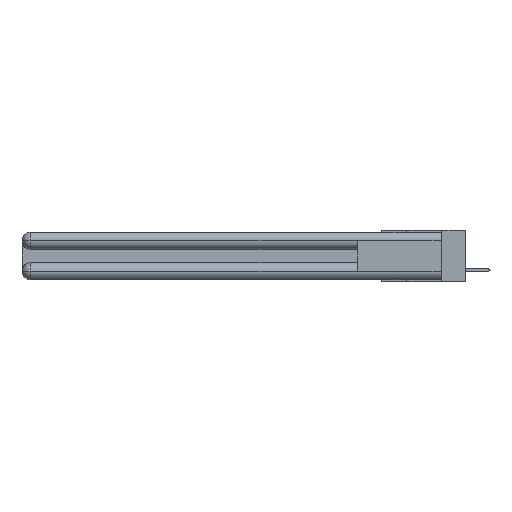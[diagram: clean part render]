
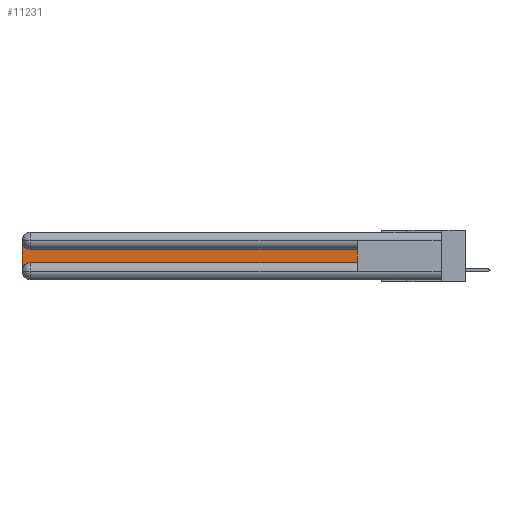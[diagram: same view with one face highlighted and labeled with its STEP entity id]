
A CAD part, left-side view. The second image highlights one B-rep face of the part: STEP entity #11231.
In plain terms, the highlighted planar face has unit normal (-1, 0, 0).
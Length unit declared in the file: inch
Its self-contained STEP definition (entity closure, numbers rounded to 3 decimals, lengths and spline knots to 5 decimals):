
#321 = ORIENTED_EDGE ( 'NONE', *, *, #31516, .T. ) ;
#532 = CARTESIAN_POINT ( 'NONE',  ( 0.075, 2.94, -0.0625 ) ) ;
#1027 = EDGE_CURVE ( 'NONE', #16137, #26790, #10930, .T. ) ;
#1420 = DIRECTION ( 'NONE',  ( 0., 1., 0. ) ) ;
#3016 = ORIENTED_EDGE ( 'NONE', *, *, #17873, .T. ) ;
#3107 = LINE ( 'NONE', #11077, #6936 ) ;
#4307 = PLANE ( 'NONE',  #23785 ) ;
#5702 = DIRECTION ( 'NONE',  ( 0., 0., 1. ) ) ;
#6268 = CARTESIAN_POINT ( 'NONE',  ( 0.075, 3., -0.2775 ) ) ;
#6413 = CARTESIAN_POINT ( 'NONE',  ( 0.075, 0.6, -0.2175 ) ) ;
#6936 = VECTOR ( 'NONE', #1420, 39.37008 ) ;
#8066 = CARTESIAN_POINT ( 'NONE',  ( 0.075, 0.6, -0.2175 ) ) ;
#8833 = EDGE_CURVE ( 'NONE', #28122, #19198, #11443, .T. ) ;
#9186 = DIRECTION ( 'NONE',  ( 1., 0., 0. ) ) ;
#9879 = ORIENTED_EDGE ( 'NONE', *, *, #1027, .T. ) ;
#9906 = AXIS2_PLACEMENT_3D ( 'NONE', #21606, #9186, #31037 ) ;
#10007 = DIRECTION ( 'NONE',  ( 1., 0., 0. ) ) ;
#10090 = CARTESIAN_POINT ( 'NONE',  ( 0.075, 0.6, -0.2175 ) ) ;
#10930 = LINE ( 'NONE', #6413, #16591 ) ;
#11077 = CARTESIAN_POINT ( 'NONE',  ( 0.075, 0.6, -0.1225 ) ) ;
#11231 = ADVANCED_FACE ( 'NONE', ( #15076 ), #4307, .F. ) ;
#11443 = LINE ( 'NONE', #30279, #20931 ) ;
#13415 = ORIENTED_EDGE ( 'NONE', *, *, #25582, .T. ) ;
#14330 = VERTEX_POINT ( 'NONE', #28066 ) ;
#15076 = FACE_OUTER_BOUND ( 'NONE', #20091, .T. ) ;
#16137 = VERTEX_POINT ( 'NONE', #19026 ) ;
#16379 = CARTESIAN_POINT ( 'NONE',  ( 0.075, 3., -0.1225 ) ) ;
#16591 = VECTOR ( 'NONE', #18416, 39.37008 ) ;
#17873 = EDGE_CURVE ( 'NONE', #26790, #30462, #20124, .T. ) ;
#17976 = DIRECTION ( 'NONE',  ( 0., 0., -1. ) ) ;
#18416 = DIRECTION ( 'NONE',  ( 0., -1., 0. ) ) ;
#18522 = EDGE_CURVE ( 'NONE', #14330, #28122, #24708, .T. ) ;
#19026 = CARTESIAN_POINT ( 'NONE',  ( 0.075, 2.94, -0.2175 ) ) ;
#19198 = VERTEX_POINT ( 'NONE', #6268 ) ;
#20091 = EDGE_LOOP ( 'NONE', ( #321, #31139, #22696, #13415, #9879, #3016 ) ) ;
#20124 = LINE ( 'NONE', #8066, #28485 ) ;
#20931 = VECTOR ( 'NONE', #17976, 39.37008 ) ;
#21606 = CARTESIAN_POINT ( 'NONE',  ( 0.075, 2.94, -0.2775 ) ) ;
#21841 = CARTESIAN_POINT ( 'NONE',  ( 0.075, 3., -0.0625 ) ) ;
#22696 = ORIENTED_EDGE ( 'NONE', *, *, #8833, .T. ) ;
#23484 = CIRCLE ( 'NONE', #9906, 0.06 ) ;
#23785 = AXIS2_PLACEMENT_3D ( 'NONE', #16379, #31264, #27937 ) ;
#24679 = AXIS2_PLACEMENT_3D ( 'NONE', #532, #10007, #27450 ) ;
#24708 = CIRCLE ( 'NONE', #24679, 0.06 ) ;
#25582 = EDGE_CURVE ( 'NONE', #19198, #16137, #23484, .T. ) ;
#26790 = VERTEX_POINT ( 'NONE', #10090 ) ;
#27450 = DIRECTION ( 'NONE',  ( 0., 0., -1. ) ) ;
#27937 = DIRECTION ( 'NONE',  ( 0., 0., -1. ) ) ;
#28066 = CARTESIAN_POINT ( 'NONE',  ( 0.075, 2.94, -0.1225 ) ) ;
#28122 = VERTEX_POINT ( 'NONE', #21841 ) ;
#28130 = CARTESIAN_POINT ( 'NONE',  ( 0.075, 0.6, -0.1225 ) ) ;
#28485 = VECTOR ( 'NONE', #5702, 39.37008 ) ;
#30279 = CARTESIAN_POINT ( 'NONE',  ( 0.075, 3., -0.2175 ) ) ;
#30462 = VERTEX_POINT ( 'NONE', #28130 ) ;
#31037 = DIRECTION ( 'NONE',  ( 0., 0., -1. ) ) ;
#31139 = ORIENTED_EDGE ( 'NONE', *, *, #18522, .T. ) ;
#31264 = DIRECTION ( 'NONE',  ( 1., 0., 0. ) ) ;
#31516 = EDGE_CURVE ( 'NONE', #30462, #14330, #3107, .T. ) ;
